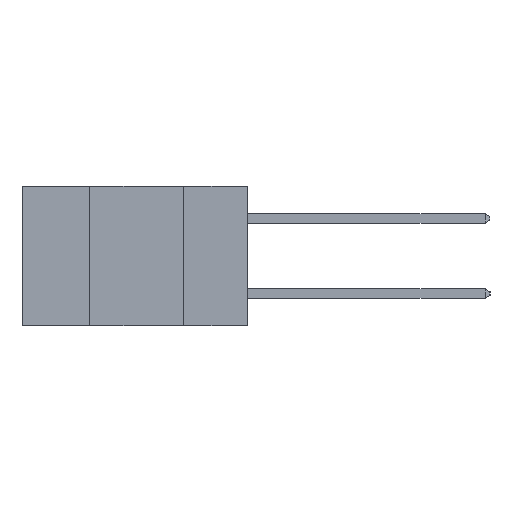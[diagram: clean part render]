
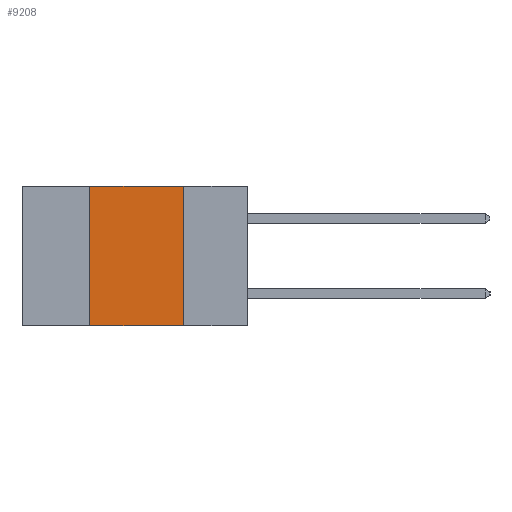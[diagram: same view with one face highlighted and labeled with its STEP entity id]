
A CAD part, left-side view. The second image highlights one B-rep face of the part: STEP entity #9208.
In plain terms, the highlighted planar face has unit normal (-1, 0, 0).
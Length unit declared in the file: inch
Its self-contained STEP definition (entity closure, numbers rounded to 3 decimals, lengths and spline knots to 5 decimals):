
#379 = LINE ( 'NONE', #764, #15558 ) ;
#764 = CARTESIAN_POINT ( 'NONE',  ( 0., 0.6, -0.37 ) ) ;
#2066 = DIRECTION ( 'NONE',  ( 0., 0., 1. ) ) ;
#2848 = DIRECTION ( 'NONE',  ( 0., -1., 0. ) ) ;
#3186 = LINE ( 'NONE', #10538, #13121 ) ;
#3913 = CARTESIAN_POINT ( 'NONE',  ( 0., 0.42, 0. ) ) ;
#4072 = CARTESIAN_POINT ( 'NONE',  ( 0., 0.42, -0.37 ) ) ;
#4620 = VERTEX_POINT ( 'NONE', #15470 ) ;
#4632 = ORIENTED_EDGE ( 'NONE', *, *, #11638, .F. ) ;
#5539 = VERTEX_POINT ( 'NONE', #3913 ) ;
#6820 = EDGE_CURVE ( 'NONE', #5539, #23735, #3186, .T. ) ;
#6824 = ORIENTED_EDGE ( 'NONE', *, *, #10220, .T. ) ;
#7129 = LINE ( 'NONE', #4072, #11768 ) ;
#9208 = ADVANCED_FACE ( 'NONE', ( #10563 ), #13216, .F. ) ;
#10220 = EDGE_CURVE ( 'NONE', #4620, #23500, #379, .T. ) ;
#10538 = CARTESIAN_POINT ( 'NONE',  ( 0., 0.6, 0. ) ) ;
#10563 = FACE_OUTER_BOUND ( 'NONE', #13622, .T. ) ;
#10687 = CARTESIAN_POINT ( 'NONE',  ( 0., 0.17, 0. ) ) ;
#10938 = ORIENTED_EDGE ( 'NONE', *, *, #21559, .F. ) ;
#11638 = EDGE_CURVE ( 'NONE', #23735, #23500, #22696, .T. ) ;
#11768 = VECTOR ( 'NONE', #2066, 39.37008 ) ;
#12077 = ORIENTED_EDGE ( 'NONE', *, *, #6820, .F. ) ;
#13100 = DIRECTION ( 'NONE',  ( 0., 0., -1. ) ) ;
#13106 = DIRECTION ( 'NONE',  ( 1., 0., 0. ) ) ;
#13121 = VECTOR ( 'NONE', #2848, 39.37008 ) ;
#13187 = CARTESIAN_POINT ( 'NONE',  ( 0., 0.6, 0. ) ) ;
#13216 = PLANE ( 'NONE',  #13892 ) ;
#13540 = DIRECTION ( 'NONE',  ( 0., 0., -1. ) ) ;
#13622 = EDGE_LOOP ( 'NONE', ( #4632, #12077, #10938, #6824 ) ) ;
#13892 = AXIS2_PLACEMENT_3D ( 'NONE', #13187, #13106, #13100 ) ;
#15470 = CARTESIAN_POINT ( 'NONE',  ( 0., 0.42, -0.37 ) ) ;
#15558 = VECTOR ( 'NONE', #22169, 39.37008 ) ;
#17637 = VECTOR ( 'NONE', #13540, 39.37008 ) ;
#17650 = CARTESIAN_POINT ( 'NONE',  ( 0., 0.17, -0.37 ) ) ;
#21559 = EDGE_CURVE ( 'NONE', #4620, #5539, #7129, .T. ) ;
#22169 = DIRECTION ( 'NONE',  ( 0., -1., 0. ) ) ;
#22696 = LINE ( 'NONE', #22994, #17637 ) ;
#22994 = CARTESIAN_POINT ( 'NONE',  ( 0., 0.17, -0.37 ) ) ;
#23500 = VERTEX_POINT ( 'NONE', #17650 ) ;
#23735 = VERTEX_POINT ( 'NONE', #10687 ) ;
